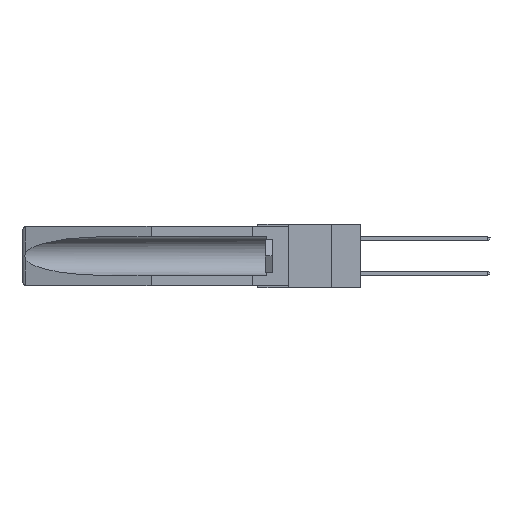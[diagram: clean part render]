
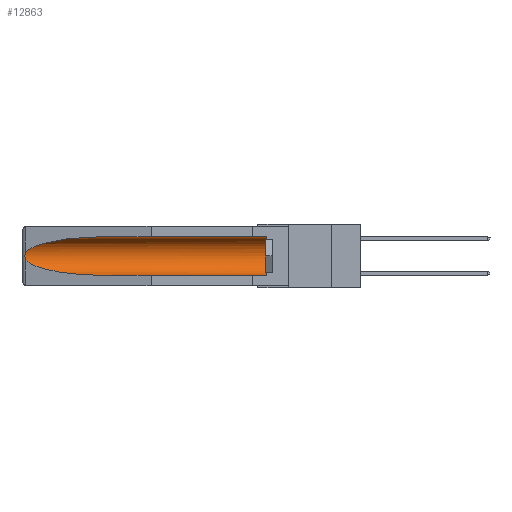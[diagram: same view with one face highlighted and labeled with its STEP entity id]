
A CAD part, left-side view. The second image highlights one B-rep face of the part: STEP entity #12863.
In plain terms, the highlighted cylindrical face has radius 2.857 mm (diameter 5.715 mm), a partial arc.
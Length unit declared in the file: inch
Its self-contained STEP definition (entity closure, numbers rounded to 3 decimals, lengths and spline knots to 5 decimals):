
#283 = DIRECTION ( 'NONE',  ( 0., 0., 1. ) ) ;
#568 = CARTESIAN_POINT ( 'NONE',  ( 0.155, 1.07973, -0.059 ) ) ;
#1393 = CARTESIAN_POINT ( 'NONE',  ( 0.155, -0.30754, -0.059 ) ) ;
#2081 = AXIS2_PLACEMENT_3D ( 'NONE', #5008, #9713, #5458 ) ;
#2237 = CARTESIAN_POINT ( 'NONE',  ( 0.26537, 1.52718, -0.19328 ) ) ;
#2382 = CARTESIAN_POINT ( 'NONE',  ( 0.155, -0.30754, -0.284 ) ) ;
#2616 = ORIENTED_EDGE ( 'NONE', *, *, #7072, .T. ) ;
#2882 = CARTESIAN_POINT ( 'NONE',  ( 0.155, 0.126, -0.059 ) ) ;
#3138 = CARTESIAN_POINT ( 'NONE',  ( 0.25451, 1.48313, -0.24835 ) ) ;
#3322 = CARTESIAN_POINT ( 'NONE',  ( 0.155, 1.07973, -0.284 ) ) ;
#4372 = ORIENTED_EDGE ( 'NONE', *, *, #11851, .T. ) ;
#4768 = CARTESIAN_POINT ( 'NONE',  ( 0.26537, 1.52718, -0.14972 ) ) ;
#5008 = CARTESIAN_POINT ( 'NONE',  ( 0.155, -0.30754, -0.1715 ) ) ;
#5124 = ORIENTED_EDGE ( 'NONE', *, *, #25786, .T. ) ;
#5458 = DIRECTION ( 'NONE',  ( 0., 0., 1. ) ) ;
#6105 = EDGE_CURVE ( 'NONE', #26543, #13344, #17830, .T. ) ;
#6167 = VECTOR ( 'NONE', #21306, 39.37008 ) ;
#6733 = CARTESIAN_POINT ( 'NONE',  ( 0.25451, 1.48313, -0.09465 ) ) ;
#6925 = CARTESIAN_POINT ( 'NONE',  ( 0.26537, 1.52718, -0.14972 ) ) ;
#7072 = EDGE_CURVE ( 'NONE', #13344, #9697, #12963, .T. ) ;
#7467 = B_SPLINE_CURVE_WITH_KNOTS ( 'NONE', 3,
 ( #26746, #7867, #24402, #8049, #16153, #22364, #11988, #16334, #14625, #2237 ),
 .UNSPECIFIED., .F., .F.,
 ( 4, 2, 2, 2, 4 ),
 ( 0., 0.00029, 0.00058, 0.00087, 0.00117 ),
 .UNSPECIFIED. ) ;
#7867 = CARTESIAN_POINT ( 'NONE',  ( 0.26597, 1.52961, -0.15275 ) ) ;
#8049 = CARTESIAN_POINT ( 'NONE',  ( 0.2673, 1.5327, -0.16383 ) ) ;
#8490 = CARTESIAN_POINT ( 'NONE',  ( 0.155, 1.07973, -0.284 ) ) ;
#9697 = VERTEX_POINT ( 'NONE', #4768 ) ;
#9713 = DIRECTION ( 'NONE',  ( 0., 1., 0. ) ) ;
#10969 = VECTOR ( 'NONE', #21055, 39.37008 ) ;
#11135 = ORIENTED_EDGE ( 'NONE', *, *, #20080, .F. ) ;
#11699 = CARTESIAN_POINT ( 'NONE',  ( 0.21114, 1.30732, -0.284 ) ) ;
#11851 = EDGE_CURVE ( 'NONE', #21336, #19498, #26688, .T. ) ;
#11988 = CARTESIAN_POINT ( 'NONE',  ( 0.2673, 1.53269, -0.17917 ) ) ;
#12863 = ADVANCED_FACE ( 'NONE', ( #15933 ), #15908, .F. ) ;
#12963 =( BOUNDED_CURVE ( )  B_SPLINE_CURVE ( 3, ( #25313, #21426, #6733, #6925 ),
 .UNSPECIFIED., .F., .F. ) 
 B_SPLINE_CURVE_WITH_KNOTS ( ( 4, 4 ),
 ( 4.71239, 6.08839 ),
 .UNSPECIFIED. ) 
 CURVE ( )  GEOMETRIC_REPRESENTATION_ITEM ( )  RATIONAL_B_SPLINE_CURVE ( ( 1., 0.848, 0.848, 1. ) ) 
 REPRESENTATION_ITEM ( '' )  );
#13082 = VERTEX_POINT ( 'NONE', #17217 ) ;
#13253 = CIRCLE ( 'NONE', #24405, 0.1125 ) ;
#13344 = VERTEX_POINT ( 'NONE', #568 ) ;
#14625 = CARTESIAN_POINT ( 'NONE',  ( 0.26597, 1.5296, -0.19026 ) ) ;
#14673 = CARTESIAN_POINT ( 'NONE',  ( 0.155, 0.126, -0.1715 ) ) ;
#14930 = EDGE_CURVE ( 'NONE', #9697, #21336, #7467, .T. ) ;
#15908 = CYLINDRICAL_SURFACE ( 'NONE', #2081, 0.1125 ) ;
#15933 = FACE_OUTER_BOUND ( 'NONE', #20237, .T. ) ;
#16153 = CARTESIAN_POINT ( 'NONE',  ( 0.2675, 1.53308, -0.16763 ) ) ;
#16334 = CARTESIAN_POINT ( 'NONE',  ( 0.26655, 1.53094, -0.18657 ) ) ;
#17083 = CARTESIAN_POINT ( 'NONE',  ( 0.26537, 1.52718, -0.19328 ) ) ;
#17217 = CARTESIAN_POINT ( 'NONE',  ( 0.155, 0.126, -0.284 ) ) ;
#17765 = ORIENTED_EDGE ( 'NONE', *, *, #14930, .T. ) ;
#17830 = LINE ( 'NONE', #1393, #6167 ) ;
#19498 = VERTEX_POINT ( 'NONE', #8490 ) ;
#20080 = EDGE_CURVE ( 'NONE', #13082, #19498, #23965, .T. ) ;
#20237 = EDGE_LOOP ( 'NONE', ( #2616, #17765, #4372, #11135, #5124, #26522 ) ) ;
#21055 = DIRECTION ( 'NONE',  ( 0., 1., 0. ) ) ;
#21306 = DIRECTION ( 'NONE',  ( 0., 1., 0. ) ) ;
#21336 = VERTEX_POINT ( 'NONE', #17083 ) ;
#21426 = CARTESIAN_POINT ( 'NONE',  ( 0.21114, 1.30732, -0.059 ) ) ;
#22364 = CARTESIAN_POINT ( 'NONE',  ( 0.2675, 1.53308, -0.17534 ) ) ;
#23965 = LINE ( 'NONE', #2382, #10969 ) ;
#24118 = CARTESIAN_POINT ( 'NONE',  ( 0.26537, 1.52718, -0.19328 ) ) ;
#24402 = CARTESIAN_POINT ( 'NONE',  ( 0.26654, 1.53092, -0.15636 ) ) ;
#24405 = AXIS2_PLACEMENT_3D ( 'NONE', #14673, #25103, #283 ) ;
#25103 = DIRECTION ( 'NONE',  ( 0., -1., 0. ) ) ;
#25313 = CARTESIAN_POINT ( 'NONE',  ( 0.155, 1.07973, -0.059 ) ) ;
#25786 = EDGE_CURVE ( 'NONE', #13082, #26543, #13253, .T. ) ;
#26522 = ORIENTED_EDGE ( 'NONE', *, *, #6105, .T. ) ;
#26543 = VERTEX_POINT ( 'NONE', #2882 ) ;
#26688 =( BOUNDED_CURVE ( )  B_SPLINE_CURVE ( 3, ( #24118, #3138, #11699, #3322 ),
 .UNSPECIFIED., .F., .F. ) 
 B_SPLINE_CURVE_WITH_KNOTS ( ( 4, 4 ),
 ( 0.1948, 1.5708 ),
 .UNSPECIFIED. ) 
 CURVE ( )  GEOMETRIC_REPRESENTATION_ITEM ( )  RATIONAL_B_SPLINE_CURVE ( ( 1., 0.848, 0.848, 1. ) ) 
 REPRESENTATION_ITEM ( '' )  );
#26746 = CARTESIAN_POINT ( 'NONE',  ( 0.26537, 1.52718, -0.14972 ) ) ;
